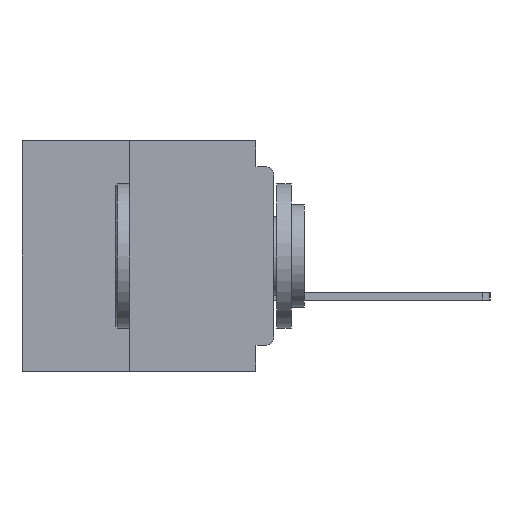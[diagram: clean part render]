
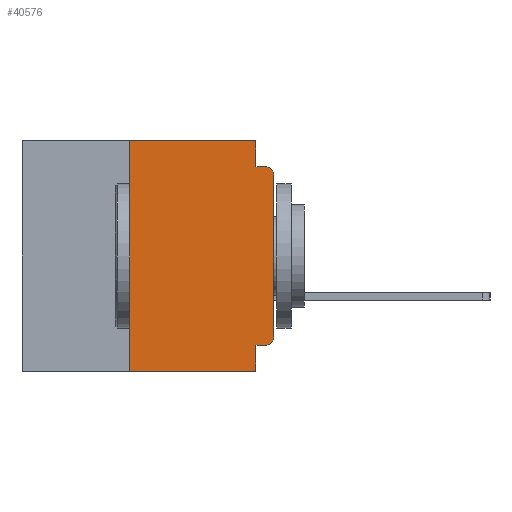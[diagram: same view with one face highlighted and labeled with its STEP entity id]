
A CAD part, left-side view. The second image highlights one B-rep face of the part: STEP entity #40576.
In plain terms, the highlighted planar face has unit normal (-1, 0, 0).
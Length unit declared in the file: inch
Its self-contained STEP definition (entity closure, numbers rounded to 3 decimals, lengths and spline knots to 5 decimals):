
#1263 = CARTESIAN_POINT ( 'NONE',  ( 0., 0., -0.355 ) ) ;
#1919 = DIRECTION ( 'NONE',  ( 0., -1., 0. ) ) ;
#1987 = VERTEX_POINT ( 'NONE', #7196 ) ;
#2530 = EDGE_CURVE ( 'NONE', #31654, #34839, #44703, .T. ) ;
#2772 = LINE ( 'NONE', #26793, #11907 ) ;
#3280 = VECTOR ( 'NONE', #45416, 39.37008 ) ;
#4222 = CARTESIAN_POINT ( 'NONE',  ( 0., 0.015, -0.355 ) ) ;
#5237 = DIRECTION ( 'NONE',  ( 0., 1., 0. ) ) ;
#5466 = EDGE_CURVE ( 'NONE', #10478, #5539, #18318, .T. ) ;
#5539 = VERTEX_POINT ( 'NONE', #30089 ) ;
#6389 = VERTEX_POINT ( 'NONE', #35915 ) ;
#6752 = ORIENTED_EDGE ( 'NONE', *, *, #49764, .F. ) ;
#7196 = CARTESIAN_POINT ( 'NONE',  ( 0., 0.031, -0.4 ) ) ;
#10478 = VERTEX_POINT ( 'NONE', #4222 ) ;
#10598 = ORIENTED_EDGE ( 'NONE', *, *, #48349, .T. ) ;
#10653 = ORIENTED_EDGE ( 'NONE', *, *, #48415, .F. ) ;
#11907 = VECTOR ( 'NONE', #50045, 39.37008 ) ;
#12323 = AXIS2_PLACEMENT_3D ( 'NONE', #48636, #37043, #13780 ) ;
#12670 = CARTESIAN_POINT ( 'NONE',  ( 0., 0.25, 0. ) ) ;
#13294 = CARTESIAN_POINT ( 'NONE',  ( 0., 0.031, 0. ) ) ;
#13780 = DIRECTION ( 'NONE',  ( 0., 0., -1. ) ) ;
#14056 = VERTEX_POINT ( 'NONE', #48326 ) ;
#14443 = DIRECTION ( 'NONE',  ( -1., 0., 0. ) ) ;
#14862 = CARTESIAN_POINT ( 'NONE',  ( 0., 0.031, 0. ) ) ;
#15514 = ORIENTED_EDGE ( 'NONE', *, *, #43839, .F. ) ;
#15761 = AXIS2_PLACEMENT_3D ( 'NONE', #45861, #22662, #49811 ) ;
#18111 = VECTOR ( 'NONE', #5237, 39.37008 ) ;
#18318 = CIRCLE ( 'NONE', #33126, 0.015 ) ;
#19729 = EDGE_CURVE ( 'NONE', #36529, #6389, #30680, .T. ) ;
#19930 = LINE ( 'NONE', #25354, #49687 ) ;
#20329 = CARTESIAN_POINT ( 'NONE',  ( 0., 0.031, -0.4 ) ) ;
#20769 = VECTOR ( 'NONE', #40459, 39.37008 ) ;
#21338 = ORIENTED_EDGE ( 'NONE', *, *, #27983, .F. ) ;
#21577 = EDGE_CURVE ( 'NONE', #5539, #36529, #36592, .T. ) ;
#22662 = DIRECTION ( 'NONE',  ( -1., 0., 0. ) ) ;
#23722 = DIRECTION ( 'NONE',  ( 0., -1., 0. ) ) ;
#24450 = ORIENTED_EDGE ( 'NONE', *, *, #2530, .F. ) ;
#24499 = EDGE_CURVE ( 'NONE', #10478, #42534, #49061, .T. ) ;
#25354 = CARTESIAN_POINT ( 'NONE',  ( 0., 0., -0.045 ) ) ;
#25405 = PLANE ( 'NONE',  #12323 ) ;
#25550 = ORIENTED_EDGE ( 'NONE', *, *, #24499, .F. ) ;
#25858 = ORIENTED_EDGE ( 'NONE', *, *, #19729, .T. ) ;
#26322 = VECTOR ( 'NONE', #27895, 39.37008 ) ;
#26793 = CARTESIAN_POINT ( 'NONE',  ( 0., 0.437, 0. ) ) ;
#27895 = DIRECTION ( 'NONE',  ( 0., 0., 1. ) ) ;
#27983 = EDGE_CURVE ( 'NONE', #34839, #44689, #2772, .T. ) ;
#29049 = ORIENTED_EDGE ( 'NONE', *, *, #21577, .T. ) ;
#30089 = CARTESIAN_POINT ( 'NONE',  ( 0., 0., -0.34 ) ) ;
#30680 = CIRCLE ( 'NONE', #15761, 0.015 ) ;
#31654 = VERTEX_POINT ( 'NONE', #36452 ) ;
#32109 = CARTESIAN_POINT ( 'NONE',  ( 0., 0., -0.06 ) ) ;
#33126 = AXIS2_PLACEMENT_3D ( 'NONE', #37684, #14443, #41572 ) ;
#34346 = CARTESIAN_POINT ( 'NONE',  ( 0., 0.031, -0.355 ) ) ;
#34839 = VERTEX_POINT ( 'NONE', #12670 ) ;
#35915 = CARTESIAN_POINT ( 'NONE',  ( 0., 0.015, -0.045 ) ) ;
#36452 = CARTESIAN_POINT ( 'NONE',  ( 0., 0.25, -0.4 ) ) ;
#36529 = VERTEX_POINT ( 'NONE', #32109 ) ;
#36592 = LINE ( 'NONE', #47215, #26322 ) ;
#37043 = DIRECTION ( 'NONE',  ( 1., 0., 0. ) ) ;
#37684 = CARTESIAN_POINT ( 'NONE',  ( 0., 0.015, -0.34 ) ) ;
#39246 = CARTESIAN_POINT ( 'NONE',  ( 0., 0.437, -0.4 ) ) ;
#39705 = ORIENTED_EDGE ( 'NONE', *, *, #5466, .T. ) ;
#40072 = LINE ( 'NONE', #20329, #48024 ) ;
#40116 = LINE ( 'NONE', #13294, #20769 ) ;
#40459 = DIRECTION ( 'NONE',  ( 0., 0., -1. ) ) ;
#40576 = ADVANCED_FACE ( 'NONE', ( #41495 ), #25405, .F. ) ;
#41463 = CARTESIAN_POINT ( 'NONE',  ( 0., 0.25, -0.4 ) ) ;
#41495 = FACE_OUTER_BOUND ( 'NONE', #48278, .T. ) ;
#41572 = DIRECTION ( 'NONE',  ( 0., 0., -1. ) ) ;
#42495 = LINE ( 'NONE', #39246, #50467 ) ;
#42534 = VERTEX_POINT ( 'NONE', #34346 ) ;
#43501 = DIRECTION ( 'NONE',  ( 0., 0., -1. ) ) ;
#43839 = EDGE_CURVE ( 'NONE', #14056, #6389, #19930, .T. ) ;
#44689 = VERTEX_POINT ( 'NONE', #14862 ) ;
#44703 = LINE ( 'NONE', #41463, #3280 ) ;
#45416 = DIRECTION ( 'NONE',  ( 0., 0., 1. ) ) ;
#45861 = CARTESIAN_POINT ( 'NONE',  ( 0., 0.015, -0.06 ) ) ;
#47215 = CARTESIAN_POINT ( 'NONE',  ( 0., 0., 0. ) ) ;
#48024 = VECTOR ( 'NONE', #43501, 39.37008 ) ;
#48278 = EDGE_LOOP ( 'NONE', ( #29049, #25858, #15514, #6752, #21338, #24450, #10598, #10653, #25550, #39705 ) ) ;
#48326 = CARTESIAN_POINT ( 'NONE',  ( 0., 0.031, -0.045 ) ) ;
#48349 = EDGE_CURVE ( 'NONE', #31654, #1987, #42495, .T. ) ;
#48415 = EDGE_CURVE ( 'NONE', #42534, #1987, #40072, .T. ) ;
#48636 = CARTESIAN_POINT ( 'NONE',  ( 0., 0.437, 0. ) ) ;
#49061 = LINE ( 'NONE', #1263, #18111 ) ;
#49687 = VECTOR ( 'NONE', #1919, 39.37008 ) ;
#49764 = EDGE_CURVE ( 'NONE', #44689, #14056, #40116, .T. ) ;
#49811 = DIRECTION ( 'NONE',  ( 0., 0., -1. ) ) ;
#50045 = DIRECTION ( 'NONE',  ( 0., -1., 0. ) ) ;
#50467 = VECTOR ( 'NONE', #23722, 39.37008 ) ;
